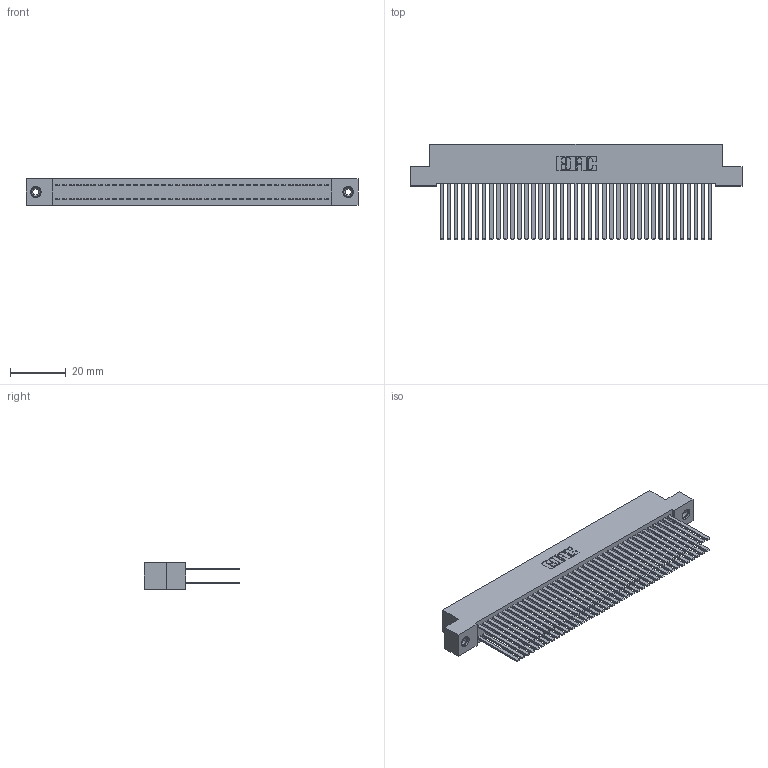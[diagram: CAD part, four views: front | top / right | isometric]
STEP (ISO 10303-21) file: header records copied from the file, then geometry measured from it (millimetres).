
FILE_DESCRIPTION (( 'STEP AP203' ), '1' );
FILE_NAME ('342-078-544-208.STEP', '2018-08-13T13:48:45', ( '' ), ( '' ), 'SwSTEP 2.0', 'SolidWorks 2016', '' );
FILE_SCHEMA (( 'CONFIG_CONTROL_DESIGN' ));
Length unit declared in the file: inch
Products named in the file (4): 342-078-544-208; 342 Part_TI; 345-292-001_345-293-144; 345-250-001_345-250-003-102
Assembly tree (81 placements, depth 2):
  342-078-544-208
    342 Part_TI
    345-292-001_345-293-144  x78
    345-250-001_345-250-003-102  x2
Bounding box: 119.38 x 34.3 x 9.4 mm (x, y, z)
Volume: 11799.8 mm3; surface area: 22171.5 mm2
Topology: 81 solids, 81 shells, 3758 faces, 11121 edges, 7302 vertices
Faces by surface type: plane 2594, cylinder 1148, cone 12, torus 4
Entity records: 26348 total; most frequent: CARTESIAN_POINT 4349, ORIENTED_EDGE 4278, DIRECTION 3749, EDGE_CURVE 2139, VECTOR 1995, LINE 1995, VERTEX_POINT 1420, AXIS2_PLACEMENT_3D 877
